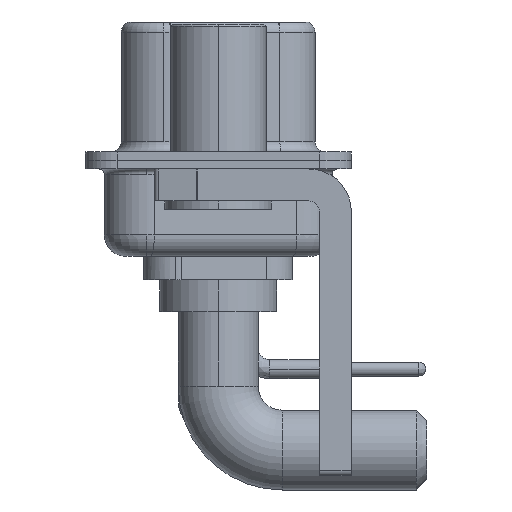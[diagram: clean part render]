
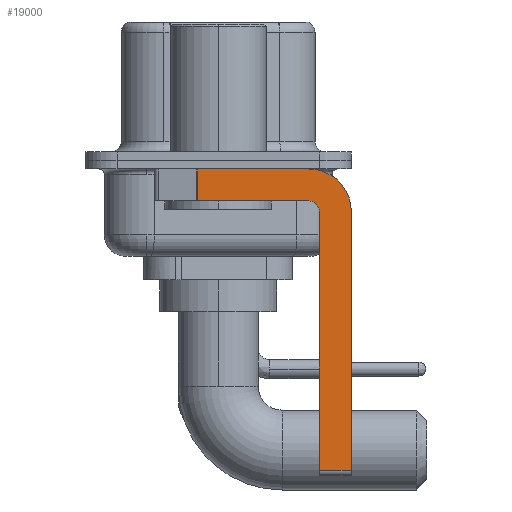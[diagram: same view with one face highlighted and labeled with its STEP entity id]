
A CAD part, left-side view. The second image highlights one B-rep face of the part: STEP entity #19000.
In plain terms, the highlighted planar face has unit normal (-1, 0, 0).
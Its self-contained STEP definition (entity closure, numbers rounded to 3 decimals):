
#1285 = EDGE_CURVE ( 'NONE', #22346, #24708, #11983, .T. ) ;
#1441 = VERTEX_POINT ( 'NONE', #19264 ) ;
#1540 = VECTOR ( 'NONE', #24788, 1000. ) ;
#1647 = PLANE ( 'NONE',  #25179 ) ;
#2329 = VERTEX_POINT ( 'NONE', #3498 ) ;
#2926 = EDGE_LOOP ( 'NONE', ( #12769, #16102, #9100, #18819, #28997, #17936, #18735, #21533 ) ) ;
#3064 = VECTOR ( 'NONE', #21267, 1000. ) ;
#3498 = CARTESIAN_POINT ( 'NONE',  ( -2.9, 0.978, -0.4 ) ) ;
#3874 = CARTESIAN_POINT ( 'NONE',  ( -2.9, -4.25, -1.9 ) ) ;
#5431 = DIRECTION ( 'NONE',  ( 0., 0., -1. ) ) ;
#5562 = EDGE_CURVE ( 'NONE', #14599, #21212, #16366, .T. ) ;
#6111 = DIRECTION ( 'NONE',  ( 0., 0., -1. ) ) ;
#6310 = AXIS2_PLACEMENT_3D ( 'NONE', #22732, #24962, #26733 ) ;
#6537 = CARTESIAN_POINT ( 'NONE',  ( -2.9, -4.75, -14.55 ) ) ;
#7427 = CARTESIAN_POINT ( 'NONE',  ( -2.9, -4.25, -0.4 ) ) ;
#7714 = CIRCLE ( 'NONE', #6310, 0.5 ) ;
#7813 = VECTOR ( 'NONE', #5431, 1000. ) ;
#9100 = ORIENTED_EDGE ( 'NONE', *, *, #1285, .F. ) ;
#9210 = VECTOR ( 'NONE', #10798, 1000. ) ;
#9575 = LINE ( 'NONE', #20699, #3064 ) ;
#9787 = CARTESIAN_POINT ( 'NONE',  ( -2.9, -4.25, -1.9 ) ) ;
#10017 = CARTESIAN_POINT ( 'NONE',  ( -2.9, -6.25, -2.4 ) ) ;
#10699 = CARTESIAN_POINT ( 'NONE',  ( -2.9, -4.25, -2.4 ) ) ;
#10798 = DIRECTION ( 'NONE',  ( 0., -1., 0. ) ) ;
#11012 = LINE ( 'NONE', #24635, #1540 ) ;
#11983 = LINE ( 'NONE', #9787, #27771 ) ;
#12181 = VERTEX_POINT ( 'NONE', #7427 ) ;
#12769 = ORIENTED_EDGE ( 'NONE', *, *, #22883, .F. ) ;
#13698 = EDGE_CURVE ( 'NONE', #21212, #22346, #7714, .T. ) ;
#14599 = VERTEX_POINT ( 'NONE', #6537 ) ;
#14741 = CARTESIAN_POINT ( 'NONE',  ( -2.9, -4.25, -2.4 ) ) ;
#15040 = DIRECTION ( 'NONE',  ( 1., 0., 0. ) ) ;
#16102 = ORIENTED_EDGE ( 'NONE', *, *, #20714, .T. ) ;
#16366 = LINE ( 'NONE', #23717, #17490 ) ;
#16465 = VERTEX_POINT ( 'NONE', #17351 ) ;
#16676 = LINE ( 'NONE', #10017, #7813 ) ;
#17229 = EDGE_CURVE ( 'NONE', #12181, #1441, #23487, .T. ) ;
#17312 = LINE ( 'NONE', #26334, #9210 ) ;
#17351 = CARTESIAN_POINT ( 'NONE',  ( -2.9, -6.25, -14.55 ) ) ;
#17490 = VECTOR ( 'NONE', #18448, 1000. ) ;
#17936 = ORIENTED_EDGE ( 'NONE', *, *, #22646, .T. ) ;
#18448 = DIRECTION ( 'NONE',  ( 0., 0., 1. ) ) ;
#18735 = ORIENTED_EDGE ( 'NONE', *, *, #22936, .F. ) ;
#18819 = ORIENTED_EDGE ( 'NONE', *, *, #13698, .F. ) ;
#18825 = DIRECTION ( 'NONE',  ( 0., 1., 0. ) ) ;
#19000 = ADVANCED_FACE ( 'NONE', ( #24161 ), #1647, .F. ) ;
#19264 = CARTESIAN_POINT ( 'NONE',  ( -2.9, -6.25, -2.4 ) ) ;
#20699 = CARTESIAN_POINT ( 'NONE',  ( -2.9, 3., -0.4 ) ) ;
#20714 = EDGE_CURVE ( 'NONE', #2329, #24708, #11012, .T. ) ;
#21212 = VERTEX_POINT ( 'NONE', #28713 ) ;
#21267 = DIRECTION ( 'NONE',  ( 0., -1., 0. ) ) ;
#21533 = ORIENTED_EDGE ( 'NONE', *, *, #17229, .F. ) ;
#22346 = VERTEX_POINT ( 'NONE', #3874 ) ;
#22543 = AXIS2_PLACEMENT_3D ( 'NONE', #14741, #15040, #24218 ) ;
#22646 = EDGE_CURVE ( 'NONE', #14599, #16465, #17312, .T. ) ;
#22732 = CARTESIAN_POINT ( 'NONE',  ( -2.9, -4.25, -2.4 ) ) ;
#22883 = EDGE_CURVE ( 'NONE', #2329, #12181, #9575, .T. ) ;
#22936 = EDGE_CURVE ( 'NONE', #1441, #16465, #16676, .T. ) ;
#23487 = CIRCLE ( 'NONE', #22543, 2. ) ;
#23717 = CARTESIAN_POINT ( 'NONE',  ( -2.9, -4.75, -14.8 ) ) ;
#24161 = FACE_OUTER_BOUND ( 'NONE', #2926, .T. ) ;
#24218 = DIRECTION ( 'NONE',  ( 0., 0., -1. ) ) ;
#24635 = CARTESIAN_POINT ( 'NONE',  ( -2.9, 0.978, -1.9 ) ) ;
#24708 = VERTEX_POINT ( 'NONE', #25068 ) ;
#24788 = DIRECTION ( 'NONE',  ( 0., 0., -1. ) ) ;
#24962 = DIRECTION ( 'NONE',  ( -1., 0., 0. ) ) ;
#25068 = CARTESIAN_POINT ( 'NONE',  ( -2.9, 0.978, -1.9 ) ) ;
#25179 = AXIS2_PLACEMENT_3D ( 'NONE', #10699, #28610, #6111 ) ;
#26334 = CARTESIAN_POINT ( 'NONE',  ( -2.9, -4.25, -14.55 ) ) ;
#26733 = DIRECTION ( 'NONE',  ( 0., 0., 1. ) ) ;
#27771 = VECTOR ( 'NONE', #18825, 1000. ) ;
#28610 = DIRECTION ( 'NONE',  ( 1., 0., 0. ) ) ;
#28713 = CARTESIAN_POINT ( 'NONE',  ( -2.9, -4.75, -2.4 ) ) ;
#28997 = ORIENTED_EDGE ( 'NONE', *, *, #5562, .F. ) ;
